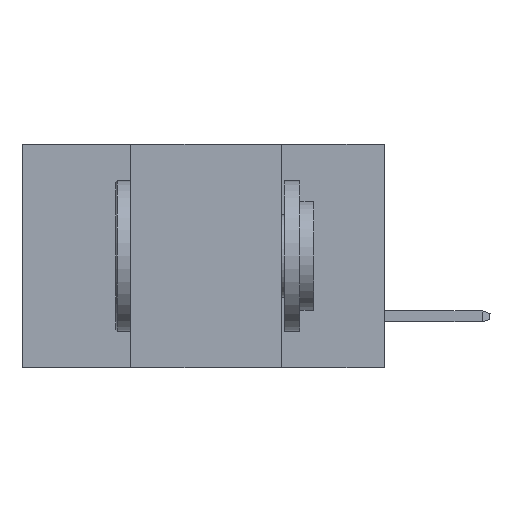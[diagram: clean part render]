
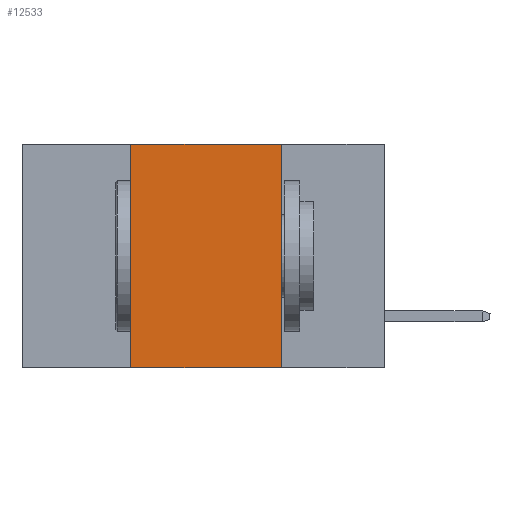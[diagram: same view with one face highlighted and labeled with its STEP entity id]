
A CAD part, left-side view. The second image highlights one B-rep face of the part: STEP entity #12533.
In plain terms, the highlighted planar face has unit normal (-1, 0, 0).
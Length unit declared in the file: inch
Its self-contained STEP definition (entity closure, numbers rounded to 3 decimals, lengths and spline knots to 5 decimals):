
#491 = LINE ( 'NONE', #12117, #632 ) ;
#632 = VECTOR ( 'NONE', #17933, 39.37008 ) ;
#712 = LINE ( 'NONE', #2225, #5005 ) ;
#756 = ORIENTED_EDGE ( 'NONE', *, *, #13140, .F. ) ;
#1606 = VERTEX_POINT ( 'NONE', #9311 ) ;
#1871 = EDGE_CURVE ( 'NONE', #7401, #5925, #8736, .T. ) ;
#2066 = CARTESIAN_POINT ( 'NONE',  ( 0., 0.17, -0.37 ) ) ;
#2225 = CARTESIAN_POINT ( 'NONE',  ( 0., 0.42, -0.37 ) ) ;
#2722 = CARTESIAN_POINT ( 'NONE',  ( 0., 0.17, 0. ) ) ;
#4188 = DIRECTION ( 'NONE',  ( 1., 0., 0. ) ) ;
#4422 = ORIENTED_EDGE ( 'NONE', *, *, #10104, .T. ) ;
#4695 = AXIS2_PLACEMENT_3D ( 'NONE', #14439, #4188, #13273 ) ;
#5005 = VECTOR ( 'NONE', #15113, 39.37008 ) ;
#5091 = EDGE_LOOP ( 'NONE', ( #14018, #6573, #756, #4422 ) ) ;
#5694 = VERTEX_POINT ( 'NONE', #12873 ) ;
#5920 = FACE_OUTER_BOUND ( 'NONE', #5091, .T. ) ;
#5925 = VERTEX_POINT ( 'NONE', #2066 ) ;
#6000 = PLANE ( 'NONE',  #4695 ) ;
#6070 = DIRECTION ( 'NONE',  ( 0., -1., 0. ) ) ;
#6573 = ORIENTED_EDGE ( 'NONE', *, *, #6690, .F. ) ;
#6690 = EDGE_CURVE ( 'NONE', #1606, #7401, #491, .T. ) ;
#7401 = VERTEX_POINT ( 'NONE', #2722 ) ;
#8473 = VECTOR ( 'NONE', #8827, 39.37008 ) ;
#8736 = LINE ( 'NONE', #18649, #8473 ) ;
#8827 = DIRECTION ( 'NONE',  ( 0., 0., -1. ) ) ;
#8857 = LINE ( 'NONE', #13331, #18070 ) ;
#9311 = CARTESIAN_POINT ( 'NONE',  ( 0., 0.42, 0. ) ) ;
#10104 = EDGE_CURVE ( 'NONE', #5694, #5925, #8857, .T. ) ;
#12117 = CARTESIAN_POINT ( 'NONE',  ( 0., 0.6, 0. ) ) ;
#12533 = ADVANCED_FACE ( 'NONE', ( #5920 ), #6000, .F. ) ;
#12873 = CARTESIAN_POINT ( 'NONE',  ( 0., 0.42, -0.37 ) ) ;
#13140 = EDGE_CURVE ( 'NONE', #5694, #1606, #712, .T. ) ;
#13273 = DIRECTION ( 'NONE',  ( 0., 0., -1. ) ) ;
#13331 = CARTESIAN_POINT ( 'NONE',  ( 0., 0.6, -0.37 ) ) ;
#14018 = ORIENTED_EDGE ( 'NONE', *, *, #1871, .F. ) ;
#14439 = CARTESIAN_POINT ( 'NONE',  ( 0., 0.6, 0. ) ) ;
#15113 = DIRECTION ( 'NONE',  ( 0., 0., 1. ) ) ;
#17933 = DIRECTION ( 'NONE',  ( 0., -1., 0. ) ) ;
#18070 = VECTOR ( 'NONE', #6070, 39.37008 ) ;
#18649 = CARTESIAN_POINT ( 'NONE',  ( 0., 0.17, -0.37 ) ) ;
